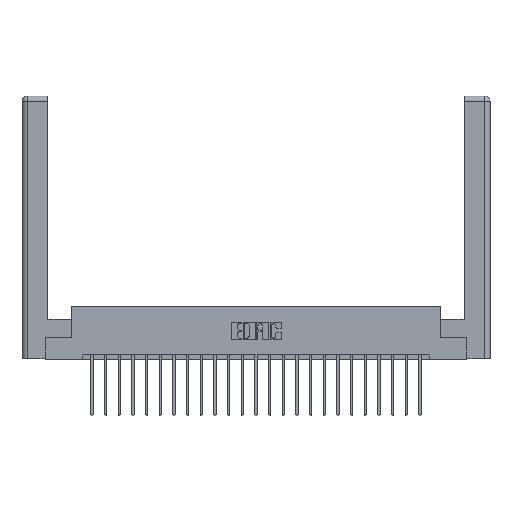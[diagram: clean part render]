
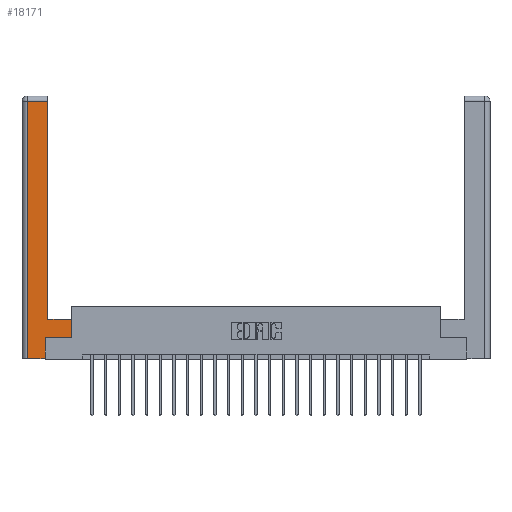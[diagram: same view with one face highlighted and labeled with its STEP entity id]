
A CAD part, top view. The second image highlights one B-rep face of the part: STEP entity #18171.
In plain terms, the highlighted planar face has unit normal (0, 0, 1).
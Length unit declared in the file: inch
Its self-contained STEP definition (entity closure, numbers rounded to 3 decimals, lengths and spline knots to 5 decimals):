
#334 = EDGE_CURVE ( 'NONE', #22184, #16907, #2866, .T. ) ;
#542 = VECTOR ( 'NONE', #20804, 39.37008 ) ;
#563 = VECTOR ( 'NONE', #5266, 39.37008 ) ;
#1451 = CARTESIAN_POINT ( 'NONE',  ( 0.295, 2.94, 0. ) ) ;
#1639 = ORIENTED_EDGE ( 'NONE', *, *, #10632, .T. ) ;
#1664 = DIRECTION ( 'NONE',  ( 0., 1., 0. ) ) ;
#2288 = VERTEX_POINT ( 'NONE', #22133 ) ;
#2390 = VECTOR ( 'NONE', #20711, 39.37008 ) ;
#2595 = CARTESIAN_POINT ( 'NONE',  ( 0.295, 0.45, 0. ) ) ;
#2620 = VERTEX_POINT ( 'NONE', #8158 ) ;
#2690 = DIRECTION ( 'NONE',  ( -1., 0., 0. ) ) ;
#2866 = LINE ( 'NONE', #21327, #11329 ) ;
#3069 = ORIENTED_EDGE ( 'NONE', *, *, #5487, .T. ) ;
#3738 = LINE ( 'NONE', #3800, #12517 ) ;
#3800 = CARTESIAN_POINT ( 'NONE',  ( 0.265, 0.245, 0. ) ) ;
#4489 = DIRECTION ( 'NONE',  ( -1., 0., 0. ) ) ;
#4577 = CARTESIAN_POINT ( 'NONE',  ( 0., 0., 0. ) ) ;
#5266 = DIRECTION ( 'NONE',  ( 0., 1., 0. ) ) ;
#5487 = EDGE_CURVE ( 'NONE', #16907, #2620, #9978, .T. ) ;
#5548 = ORIENTED_EDGE ( 'NONE', *, *, #14916, .T. ) ;
#5665 = CARTESIAN_POINT ( 'NONE',  ( 0.265, 0., 0. ) ) ;
#6590 = VERTEX_POINT ( 'NONE', #13423 ) ;
#8116 = LINE ( 'NONE', #15038, #542 ) ;
#8158 = CARTESIAN_POINT ( 'NONE',  ( 0.0615, 0., 0. ) ) ;
#8202 = ORIENTED_EDGE ( 'NONE', *, *, #12779, .T. ) ;
#8846 = CARTESIAN_POINT ( 'NONE',  ( 0.0615, 0., 0. ) ) ;
#9978 = LINE ( 'NONE', #8846, #13768 ) ;
#10312 = LINE ( 'NONE', #5665, #2390 ) ;
#10448 = EDGE_LOOP ( 'NONE', ( #1639, #13562, #3069, #8202, #16269, #18637, #15269, #5548 ) ) ;
#10632 = EDGE_CURVE ( 'NONE', #13021, #22184, #17128, .T. ) ;
#11329 = VECTOR ( 'NONE', #2690, 39.37008 ) ;
#11922 = CARTESIAN_POINT ( 'NONE',  ( 0.265, 0., 0. ) ) ;
#11937 = LINE ( 'NONE', #12863, #563 ) ;
#12137 = AXIS2_PLACEMENT_3D ( 'NONE', #4577, #13817, #4489 ) ;
#12517 = VECTOR ( 'NONE', #16930, 39.37008 ) ;
#12595 = DIRECTION ( 'NONE',  ( 0., -1., 0. ) ) ;
#12664 = CARTESIAN_POINT ( 'NONE',  ( 0.295, 3., 0. ) ) ;
#12779 = EDGE_CURVE ( 'NONE', #2620, #17870, #10312, .T. ) ;
#12863 = CARTESIAN_POINT ( 'NONE',  ( 0.565, 0.45, 0. ) ) ;
#13021 = VERTEX_POINT ( 'NONE', #2595 ) ;
#13423 = CARTESIAN_POINT ( 'NONE',  ( 0.565, 0.245, 0. ) ) ;
#13562 = ORIENTED_EDGE ( 'NONE', *, *, #334, .T. ) ;
#13768 = VECTOR ( 'NONE', #12595, 39.37008 ) ;
#13817 = DIRECTION ( 'NONE',  ( 0., 0., -1. ) ) ;
#13822 = DIRECTION ( 'NONE',  ( -1., 0., 0. ) ) ;
#13863 = VECTOR ( 'NONE', #1664, 39.37008 ) ;
#14916 = EDGE_CURVE ( 'NONE', #23165, #13021, #20489, .T. ) ;
#15038 = CARTESIAN_POINT ( 'NONE',  ( 0.565, 0.245, 0. ) ) ;
#15269 = ORIENTED_EDGE ( 'NONE', *, *, #17529, .T. ) ;
#15491 = VECTOR ( 'NONE', #13822, 39.37008 ) ;
#16269 = ORIENTED_EDGE ( 'NONE', *, *, #17564, .T. ) ;
#16907 = VERTEX_POINT ( 'NONE', #18858 ) ;
#16930 = DIRECTION ( 'NONE',  ( 0., 1., 0. ) ) ;
#17128 = LINE ( 'NONE', #12664, #13863 ) ;
#17529 = EDGE_CURVE ( 'NONE', #6590, #23165, #11937, .T. ) ;
#17564 = EDGE_CURVE ( 'NONE', #17870, #2288, #3738, .T. ) ;
#17588 = EDGE_CURVE ( 'NONE', #2288, #6590, #8116, .T. ) ;
#17870 = VERTEX_POINT ( 'NONE', #11922 ) ;
#18171 = ADVANCED_FACE ( 'NONE', ( #19590 ), #23208, .F. ) ;
#18637 = ORIENTED_EDGE ( 'NONE', *, *, #17588, .T. ) ;
#18858 = CARTESIAN_POINT ( 'NONE',  ( 0.0615, 2.94, 0. ) ) ;
#19590 = FACE_OUTER_BOUND ( 'NONE', #10448, .T. ) ;
#19671 = CARTESIAN_POINT ( 'NONE',  ( 0.565, 0.45, 0. ) ) ;
#20489 = LINE ( 'NONE', #21338, #15491 ) ;
#20711 = DIRECTION ( 'NONE',  ( 1., 0., 0. ) ) ;
#20804 = DIRECTION ( 'NONE',  ( 1., 0., 0. ) ) ;
#21327 = CARTESIAN_POINT ( 'NONE',  ( 0.0615, 2.94, 0. ) ) ;
#21338 = CARTESIAN_POINT ( 'NONE',  ( 0.295, 0.45, 0. ) ) ;
#22133 = CARTESIAN_POINT ( 'NONE',  ( 0.265, 0.245, 0. ) ) ;
#22184 = VERTEX_POINT ( 'NONE', #1451 ) ;
#23165 = VERTEX_POINT ( 'NONE', #19671 ) ;
#23208 = PLANE ( 'NONE',  #12137 ) ;
